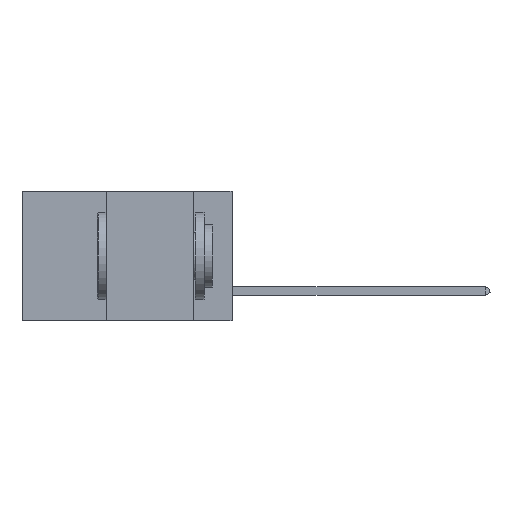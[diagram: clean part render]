
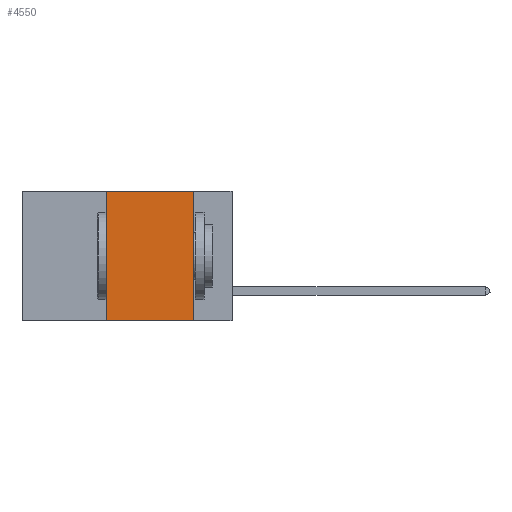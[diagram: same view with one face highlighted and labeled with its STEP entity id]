
A CAD part, left-side view. The second image highlights one B-rep face of the part: STEP entity #4550.
In plain terms, the highlighted planar face has unit normal (-1, 0, 0).
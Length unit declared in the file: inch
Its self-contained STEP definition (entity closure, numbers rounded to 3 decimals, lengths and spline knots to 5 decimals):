
#717 = CARTESIAN_POINT ( 'NONE',  ( 0., 0.11, 0. ) ) ;
#789 = DIRECTION ( 'NONE',  ( 0., 0., 1. ) ) ;
#2369 = CARTESIAN_POINT ( 'NONE',  ( 0., 0.36, -0.37 ) ) ;
#2601 = EDGE_CURVE ( 'NONE', #12655, #18052, #6566, .T. ) ;
#3657 = FACE_OUTER_BOUND ( 'NONE', #8714, .T. ) ;
#3942 = LINE ( 'NONE', #6289, #8003 ) ;
#4343 = DIRECTION ( 'NONE',  ( 0., -1., 0. ) ) ;
#4550 = ADVANCED_FACE ( 'NONE', ( #3657 ), #9687, .F. ) ;
#4749 = CARTESIAN_POINT ( 'NONE',  ( 0., 0.11, -0.37 ) ) ;
#4966 = ORIENTED_EDGE ( 'NONE', *, *, #2601, .F. ) ;
#5855 = EDGE_CURVE ( 'NONE', #20224, #18685, #15011, .T. ) ;
#6030 = VECTOR ( 'NONE', #12833, 39.37008 ) ;
#6289 = CARTESIAN_POINT ( 'NONE',  ( 0., 0.6, -0.37 ) ) ;
#6566 = LINE ( 'NONE', #717, #6030 ) ;
#7944 = CARTESIAN_POINT ( 'NONE',  ( 0., 0.6, 0. ) ) ;
#8003 = VECTOR ( 'NONE', #21869, 39.37008 ) ;
#8461 = EDGE_CURVE ( 'NONE', #18685, #12655, #10488, .T. ) ;
#8714 = EDGE_LOOP ( 'NONE', ( #4966, #12926, #12134, #11586 ) ) ;
#9259 = CARTESIAN_POINT ( 'NONE',  ( 0., 0.6, 0. ) ) ;
#9687 = PLANE ( 'NONE',  #18950 ) ;
#10362 = VECTOR ( 'NONE', #789, 39.37008 ) ;
#10488 = LINE ( 'NONE', #9259, #12945 ) ;
#11464 = DIRECTION ( 'NONE',  ( 1., 0., 0. ) ) ;
#11472 = CARTESIAN_POINT ( 'NONE',  ( 0., 0.36, 0. ) ) ;
#11586 = ORIENTED_EDGE ( 'NONE', *, *, #11838, .T. ) ;
#11838 = EDGE_CURVE ( 'NONE', #20224, #18052, #3942, .T. ) ;
#12134 = ORIENTED_EDGE ( 'NONE', *, *, #5855, .F. ) ;
#12655 = VERTEX_POINT ( 'NONE', #20147 ) ;
#12833 = DIRECTION ( 'NONE',  ( 0., 0., -1. ) ) ;
#12926 = ORIENTED_EDGE ( 'NONE', *, *, #8461, .F. ) ;
#12945 = VECTOR ( 'NONE', #4343, 39.37008 ) ;
#13205 = DIRECTION ( 'NONE',  ( 0., 0., -1. ) ) ;
#15011 = LINE ( 'NONE', #11472, #10362 ) ;
#15492 = CARTESIAN_POINT ( 'NONE',  ( 0., 0.36, 0. ) ) ;
#18052 = VERTEX_POINT ( 'NONE', #4749 ) ;
#18685 = VERTEX_POINT ( 'NONE', #15492 ) ;
#18950 = AXIS2_PLACEMENT_3D ( 'NONE', #7944, #11464, #13205 ) ;
#20147 = CARTESIAN_POINT ( 'NONE',  ( 0., 0.11, 0. ) ) ;
#20224 = VERTEX_POINT ( 'NONE', #2369 ) ;
#21869 = DIRECTION ( 'NONE',  ( 0., -1., 0. ) ) ;
